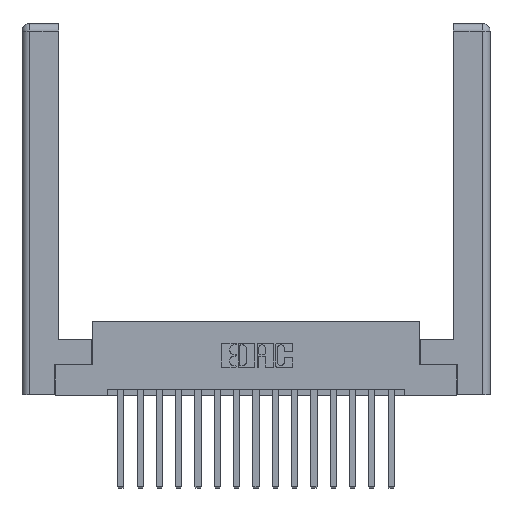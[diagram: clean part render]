
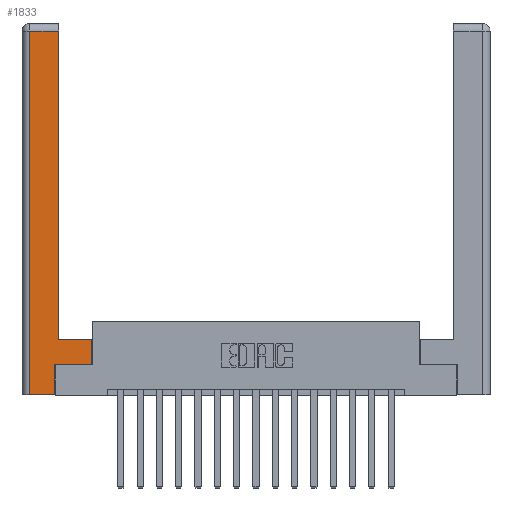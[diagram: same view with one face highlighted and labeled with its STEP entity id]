
A CAD part, top view. The second image highlights one B-rep face of the part: STEP entity #1833.
In plain terms, the highlighted planar face has unit normal (0, 0, 1).
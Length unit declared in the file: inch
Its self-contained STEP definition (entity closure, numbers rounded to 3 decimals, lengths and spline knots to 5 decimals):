
#58 = VECTOR ( 'NONE', #11922, 39.37008 ) ;
#115 = CARTESIAN_POINT ( 'NONE',  ( 0.0615, 0., 0. ) ) ;
#289 = LINE ( 'NONE', #13397, #15413 ) ;
#409 = VECTOR ( 'NONE', #8629, 39.37008 ) ;
#536 = LINE ( 'NONE', #6232, #8604 ) ;
#634 = LINE ( 'NONE', #15552, #7437 ) ;
#726 = PLANE ( 'NONE',  #1716 ) ;
#925 = LINE ( 'NONE', #9366, #3675 ) ;
#947 = ORIENTED_EDGE ( 'NONE', *, *, #15883, .T. ) ;
#960 = VERTEX_POINT ( 'NONE', #15069 ) ;
#1008 = ORIENTED_EDGE ( 'NONE', *, *, #16150, .T. ) ;
#1593 = VECTOR ( 'NONE', #6943, 39.37008 ) ;
#1716 = AXIS2_PLACEMENT_3D ( 'NONE', #7617, #11588, #3456 ) ;
#1803 = LINE ( 'NONE', #9435, #1593 ) ;
#1833 = ADVANCED_FACE ( 'NONE', ( #3837 ), #726, .F. ) ;
#2296 = CARTESIAN_POINT ( 'NONE',  ( 0.565, 0.245, 0. ) ) ;
#3456 = DIRECTION ( 'NONE',  ( -1., 0., 0. ) ) ;
#3675 = VECTOR ( 'NONE', #9539, 39.37008 ) ;
#3814 = ORIENTED_EDGE ( 'NONE', *, *, #13183, .T. ) ;
#3818 = EDGE_CURVE ( 'NONE', #16114, #10120, #536, .T. ) ;
#3837 = FACE_OUTER_BOUND ( 'NONE', #4201, .T. ) ;
#4099 = VERTEX_POINT ( 'NONE', #16164 ) ;
#4146 = EDGE_CURVE ( 'NONE', #10120, #6320, #1803, .T. ) ;
#4201 = EDGE_LOOP ( 'NONE', ( #15344, #8737, #13030, #3814, #15491, #947, #7567, #1008 ) ) ;
#4712 = LINE ( 'NONE', #6288, #58 ) ;
#6006 = EDGE_CURVE ( 'NONE', #960, #10307, #289, .T. ) ;
#6232 = CARTESIAN_POINT ( 'NONE',  ( 0.0615, 2.94, 0. ) ) ;
#6288 = CARTESIAN_POINT ( 'NONE',  ( 0.265, 0., 0. ) ) ;
#6320 = VERTEX_POINT ( 'NONE', #115 ) ;
#6440 = EDGE_CURVE ( 'NONE', #15701, #13265, #925, .T. ) ;
#6905 = CARTESIAN_POINT ( 'NONE',  ( 0.0615, 2.94, 0. ) ) ;
#6943 = DIRECTION ( 'NONE',  ( 0., -1., 0. ) ) ;
#7224 = CARTESIAN_POINT ( 'NONE',  ( 0.265, 0.245, 0. ) ) ;
#7437 = VECTOR ( 'NONE', #11608, 39.37008 ) ;
#7567 = ORIENTED_EDGE ( 'NONE', *, *, #6440, .T. ) ;
#7617 = CARTESIAN_POINT ( 'NONE',  ( 0., 0., 0. ) ) ;
#8604 = VECTOR ( 'NONE', #14443, 39.37008 ) ;
#8629 = DIRECTION ( 'NONE',  ( -1., 0., 0. ) ) ;
#8737 = ORIENTED_EDGE ( 'NONE', *, *, #3818, .T. ) ;
#9366 = CARTESIAN_POINT ( 'NONE',  ( 0.565, 0.45, 0. ) ) ;
#9435 = CARTESIAN_POINT ( 'NONE',  ( 0.0615, 0., 0. ) ) ;
#9527 = LINE ( 'NONE', #13500, #12074 ) ;
#9539 = DIRECTION ( 'NONE',  ( 0., 1., 0. ) ) ;
#10120 = VERTEX_POINT ( 'NONE', #6905 ) ;
#10307 = VERTEX_POINT ( 'NONE', #7224 ) ;
#10918 = CARTESIAN_POINT ( 'NONE',  ( 0.565, 0.45, 0. ) ) ;
#11588 = DIRECTION ( 'NONE',  ( 0., 0., -1. ) ) ;
#11608 = DIRECTION ( 'NONE',  ( 0., 1., 0. ) ) ;
#11922 = DIRECTION ( 'NONE',  ( 1., 0., 0. ) ) ;
#12074 = VECTOR ( 'NONE', #12129, 39.37008 ) ;
#12129 = DIRECTION ( 'NONE',  ( 1., 0., 0. ) ) ;
#13030 = ORIENTED_EDGE ( 'NONE', *, *, #4146, .T. ) ;
#13183 = EDGE_CURVE ( 'NONE', #6320, #960, #4712, .T. ) ;
#13265 = VERTEX_POINT ( 'NONE', #10918 ) ;
#13397 = CARTESIAN_POINT ( 'NONE',  ( 0.265, 0.245, 0. ) ) ;
#13500 = CARTESIAN_POINT ( 'NONE',  ( 0.565, 0.245, 0. ) ) ;
#14443 = DIRECTION ( 'NONE',  ( -1., 0., 0. ) ) ;
#15069 = CARTESIAN_POINT ( 'NONE',  ( 0.265, 0., 0. ) ) ;
#15184 = CARTESIAN_POINT ( 'NONE',  ( 0.295, 2.94, 0. ) ) ;
#15344 = ORIENTED_EDGE ( 'NONE', *, *, #15664, .T. ) ;
#15413 = VECTOR ( 'NONE', #17569, 39.37008 ) ;
#15491 = ORIENTED_EDGE ( 'NONE', *, *, #6006, .T. ) ;
#15497 = LINE ( 'NONE', #16773, #409 ) ;
#15552 = CARTESIAN_POINT ( 'NONE',  ( 0.295, 3., 0. ) ) ;
#15664 = EDGE_CURVE ( 'NONE', #4099, #16114, #634, .T. ) ;
#15701 = VERTEX_POINT ( 'NONE', #2296 ) ;
#15883 = EDGE_CURVE ( 'NONE', #10307, #15701, #9527, .T. ) ;
#16114 = VERTEX_POINT ( 'NONE', #15184 ) ;
#16150 = EDGE_CURVE ( 'NONE', #13265, #4099, #15497, .T. ) ;
#16164 = CARTESIAN_POINT ( 'NONE',  ( 0.295, 0.45, 0. ) ) ;
#16773 = CARTESIAN_POINT ( 'NONE',  ( 0.295, 0.45, 0. ) ) ;
#17569 = DIRECTION ( 'NONE',  ( 0., 1., 0. ) ) ;
